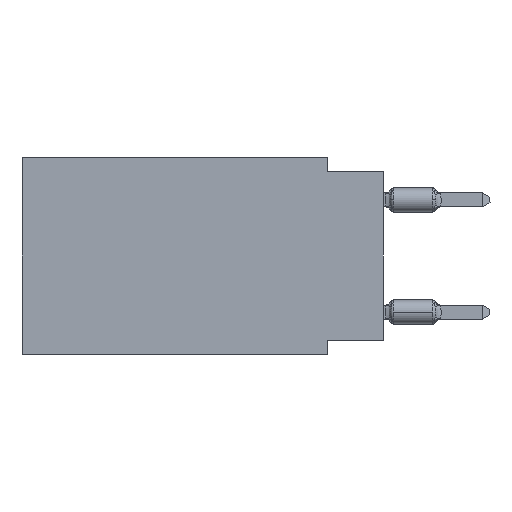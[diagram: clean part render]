
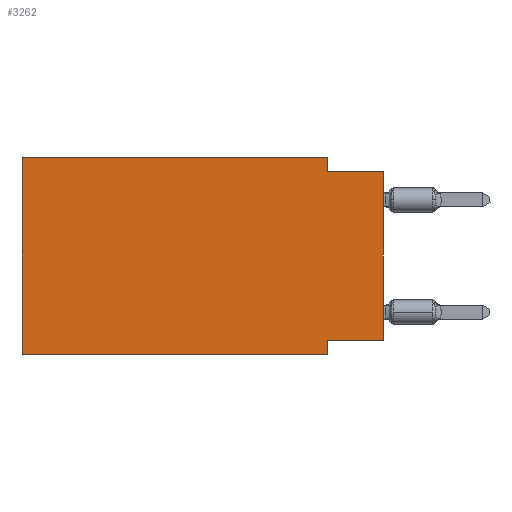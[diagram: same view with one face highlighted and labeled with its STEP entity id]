
A CAD part, left-side view. The second image highlights one B-rep face of the part: STEP entity #3262.
In plain terms, the highlighted planar face has unit normal (-1, 0, 0).
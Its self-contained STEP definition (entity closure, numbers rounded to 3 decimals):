
#418 = CARTESIAN_POINT ( 'NONE',  ( 0., 2.54, -8.255 ) ) ;
#656 = VECTOR ( 'NONE', #8381, 1000. ) ;
#725 = CARTESIAN_POINT ( 'NONE',  ( 0., 2.54, -0.635 ) ) ;
#773 = VECTOR ( 'NONE', #3780, 1000. ) ;
#819 = DIRECTION ( 'NONE',  ( 1., 0., 0. ) ) ;
#1377 = VERTEX_POINT ( 'NONE', #10769 ) ;
#1806 = VERTEX_POINT ( 'NONE', #9603 ) ;
#1966 = VERTEX_POINT ( 'NONE', #13024 ) ;
#1970 = DIRECTION ( 'NONE',  ( 0., 0., 1. ) ) ;
#2068 = CARTESIAN_POINT ( 'NONE',  ( 0., 16.383, 0. ) ) ;
#2430 = CARTESIAN_POINT ( 'NONE',  ( 0., 16.383, 0. ) ) ;
#2550 = ORIENTED_EDGE ( 'NONE', *, *, #13471, .F. ) ;
#3168 = LINE ( 'NONE', #10648, #8796 ) ;
#3262 = ADVANCED_FACE ( 'NONE', ( #16263 ), #13828, .F. ) ;
#3780 = DIRECTION ( 'NONE',  ( 0., 0., 1. ) ) ;
#3818 = VERTEX_POINT ( 'NONE', #16748 ) ;
#3857 = CARTESIAN_POINT ( 'NONE',  ( 0., 2.54, 0. ) ) ;
#4051 = VECTOR ( 'NONE', #8105, 1000. ) ;
#4242 = EDGE_LOOP ( 'NONE', ( #11779, #14372, #7622, #2550, #11570, #9637, #9006, #13843 ) ) ;
#4677 = LINE ( 'NONE', #7235, #12344 ) ;
#4679 = CARTESIAN_POINT ( 'NONE',  ( 0., 0., 0. ) ) ;
#5575 = CARTESIAN_POINT ( 'NONE',  ( 0., 16.383, -8.89 ) ) ;
#6663 = EDGE_CURVE ( 'NONE', #3818, #1377, #15144, .T. ) ;
#7235 = CARTESIAN_POINT ( 'NONE',  ( 0., 2.54, -8.89 ) ) ;
#7622 = ORIENTED_EDGE ( 'NONE', *, *, #13704, .F. ) ;
#8105 = DIRECTION ( 'NONE',  ( 0., -1., 0. ) ) ;
#8381 = DIRECTION ( 'NONE',  ( 0., 1., 0. ) ) ;
#8796 = VECTOR ( 'NONE', #10824, 1000. ) ;
#9006 = ORIENTED_EDGE ( 'NONE', *, *, #13827, .F. ) ;
#9379 = LINE ( 'NONE', #14478, #4051 ) ;
#9446 = VECTOR ( 'NONE', #10664, 1000. ) ;
#9603 = CARTESIAN_POINT ( 'NONE',  ( 0., 2.54, -8.89 ) ) ;
#9637 = ORIENTED_EDGE ( 'NONE', *, *, #12011, .T. ) ;
#9733 = LINE ( 'NONE', #14847, #656 ) ;
#9755 = VERTEX_POINT ( 'NONE', #3857 ) ;
#10648 = CARTESIAN_POINT ( 'NONE',  ( 0., 2.54, 0. ) ) ;
#10664 = DIRECTION ( 'NONE',  ( 0., -1., 0. ) ) ;
#10769 = CARTESIAN_POINT ( 'NONE',  ( 0., 0., -0.635 ) ) ;
#10784 = VERTEX_POINT ( 'NONE', #418 ) ;
#10787 = EDGE_CURVE ( 'NONE', #3818, #10784, #9733, .T. ) ;
#10824 = DIRECTION ( 'NONE',  ( 0., 0., -1. ) ) ;
#11337 = LINE ( 'NONE', #2430, #11797 ) ;
#11570 = ORIENTED_EDGE ( 'NONE', *, *, #12420, .F. ) ;
#11779 = ORIENTED_EDGE ( 'NONE', *, *, #6663, .T. ) ;
#11797 = VECTOR ( 'NONE', #16510, 1000. ) ;
#12011 = EDGE_CURVE ( 'NONE', #1966, #1806, #15936, .T. ) ;
#12344 = VECTOR ( 'NONE', #13695, 1000. ) ;
#12420 = EDGE_CURVE ( 'NONE', #1966, #15715, #15414, .T. ) ;
#12540 = DIRECTION ( 'NONE',  ( 0., 0., -1. ) ) ;
#12553 = EDGE_CURVE ( 'NONE', #13413, #1377, #9379, .T. ) ;
#13024 = CARTESIAN_POINT ( 'NONE',  ( 0., 16.383, -8.89 ) ) ;
#13413 = VERTEX_POINT ( 'NONE', #725 ) ;
#13471 = EDGE_CURVE ( 'NONE', #15715, #9755, #11337, .T. ) ;
#13474 = VECTOR ( 'NONE', #1970, 1000. ) ;
#13695 = DIRECTION ( 'NONE',  ( 0., 0., -1. ) ) ;
#13704 = EDGE_CURVE ( 'NONE', #9755, #13413, #3168, .T. ) ;
#13827 = EDGE_CURVE ( 'NONE', #10784, #1806, #4677, .T. ) ;
#13828 = PLANE ( 'NONE',  #16004 ) ;
#13843 = ORIENTED_EDGE ( 'NONE', *, *, #10787, .F. ) ;
#14322 = CARTESIAN_POINT ( 'NONE',  ( 0., 16.383, 0. ) ) ;
#14372 = ORIENTED_EDGE ( 'NONE', *, *, #12553, .F. ) ;
#14478 = CARTESIAN_POINT ( 'NONE',  ( 0., 0., -0.635 ) ) ;
#14847 = CARTESIAN_POINT ( 'NONE',  ( 0., 0., -8.255 ) ) ;
#15144 = LINE ( 'NONE', #4679, #13474 ) ;
#15414 = LINE ( 'NONE', #14322, #773 ) ;
#15715 = VERTEX_POINT ( 'NONE', #2068 ) ;
#15936 = LINE ( 'NONE', #5575, #9446 ) ;
#16004 = AXIS2_PLACEMENT_3D ( 'NONE', #16101, #819, #12540 ) ;
#16101 = CARTESIAN_POINT ( 'NONE',  ( 0., 16.383, 0. ) ) ;
#16263 = FACE_OUTER_BOUND ( 'NONE', #4242, .T. ) ;
#16510 = DIRECTION ( 'NONE',  ( 0., -1., 0. ) ) ;
#16748 = CARTESIAN_POINT ( 'NONE',  ( 0., 0., -8.255 ) ) ;
